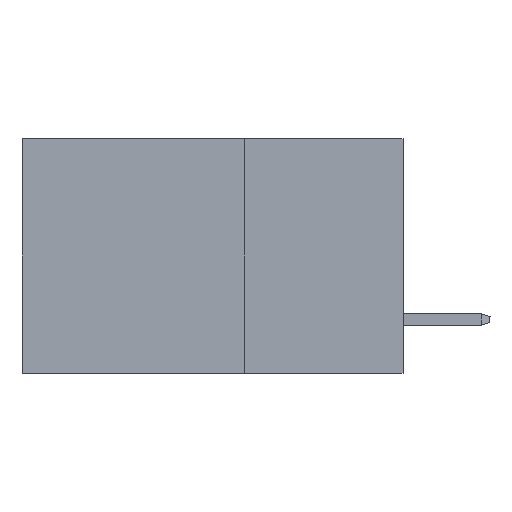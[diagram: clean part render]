
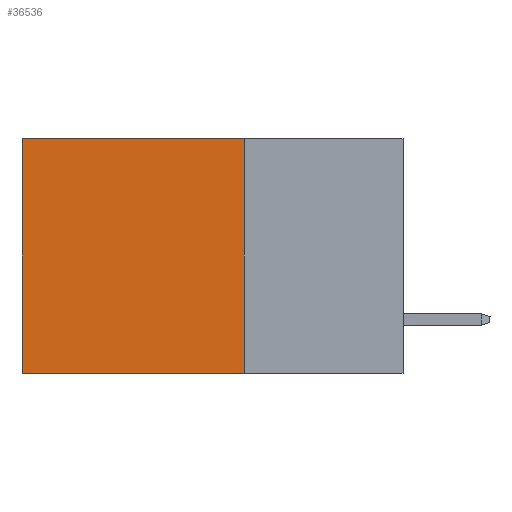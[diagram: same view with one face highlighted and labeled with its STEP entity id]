
A CAD part, left-side view. The second image highlights one B-rep face of the part: STEP entity #36536.
In plain terms, the highlighted planar face has unit normal (-1, 0, 0).
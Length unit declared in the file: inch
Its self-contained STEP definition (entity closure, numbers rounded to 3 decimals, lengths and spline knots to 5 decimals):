
#1917 = ORIENTED_EDGE ( 'NONE', *, *, #36178, .T. ) ;
#2450 = LINE ( 'NONE', #32390, #39611 ) ;
#3340 = VERTEX_POINT ( 'NONE', #43664 ) ;
#3803 = FACE_OUTER_BOUND ( 'NONE', #22108, .T. ) ;
#7436 = CARTESIAN_POINT ( 'NONE',  ( 0.2875, 0.25, 0. ) ) ;
#9761 = ORIENTED_EDGE ( 'NONE', *, *, #46366, .F. ) ;
#10947 = EDGE_CURVE ( 'NONE', #3340, #27607, #27622, .T. ) ;
#12182 = CARTESIAN_POINT ( 'NONE',  ( 0.2875, 0.25, -0.37 ) ) ;
#12780 = VECTOR ( 'NONE', #21693, 39.37008 ) ;
#13102 = DIRECTION ( 'NONE',  ( 0., 0., -1. ) ) ;
#13595 = VERTEX_POINT ( 'NONE', #14378 ) ;
#14232 = LINE ( 'NONE', #28940, #12780 ) ;
#14378 = CARTESIAN_POINT ( 'NONE',  ( 0.2875, 0.25, 0. ) ) ;
#15356 = ORIENTED_EDGE ( 'NONE', *, *, #10947, .F. ) ;
#18044 = AXIS2_PLACEMENT_3D ( 'NONE', #7436, #22864, #22143 ) ;
#20188 = DIRECTION ( 'NONE',  ( 0., 1., 0. ) ) ;
#21693 = DIRECTION ( 'NONE',  ( 0., 0., -1. ) ) ;
#22108 = EDGE_LOOP ( 'NONE', ( #26360, #15356, #9761, #1917 ) ) ;
#22143 = DIRECTION ( 'NONE',  ( 0., 0., -1. ) ) ;
#22864 = DIRECTION ( 'NONE',  ( 1., 0., 0. ) ) ;
#26360 = ORIENTED_EDGE ( 'NONE', *, *, #39595, .T. ) ;
#27607 = VERTEX_POINT ( 'NONE', #42770 ) ;
#27622 = LINE ( 'NONE', #12182, #44664 ) ;
#28940 = CARTESIAN_POINT ( 'NONE',  ( 0.2875, 0.6, 0. ) ) ;
#29472 = VERTEX_POINT ( 'NONE', #36839 ) ;
#31011 = DIRECTION ( 'NONE',  ( 0., 1., 0. ) ) ;
#32390 = CARTESIAN_POINT ( 'NONE',  ( 0.2875, 0.25, 0. ) ) ;
#36178 = EDGE_CURVE ( 'NONE', #13595, #29472, #2450, .T. ) ;
#36536 = ADVANCED_FACE ( 'NONE', ( #3803 ), #40776, .F. ) ;
#36839 = CARTESIAN_POINT ( 'NONE',  ( 0.2875, 0.6, 0. ) ) ;
#39595 = EDGE_CURVE ( 'NONE', #29472, #27607, #14232, .T. ) ;
#39611 = VECTOR ( 'NONE', #20188, 39.37008 ) ;
#40776 = PLANE ( 'NONE',  #18044 ) ;
#42770 = CARTESIAN_POINT ( 'NONE',  ( 0.2875, 0.6, -0.37 ) ) ;
#42814 = LINE ( 'NONE', #46185, #46354 ) ;
#43664 = CARTESIAN_POINT ( 'NONE',  ( 0.2875, 0.25, -0.37 ) ) ;
#44664 = VECTOR ( 'NONE', #31011, 39.37008 ) ;
#46185 = CARTESIAN_POINT ( 'NONE',  ( 0.2875, 0.25, 0. ) ) ;
#46354 = VECTOR ( 'NONE', #13102, 39.37008 ) ;
#46366 = EDGE_CURVE ( 'NONE', #13595, #3340, #42814, .T. ) ;
